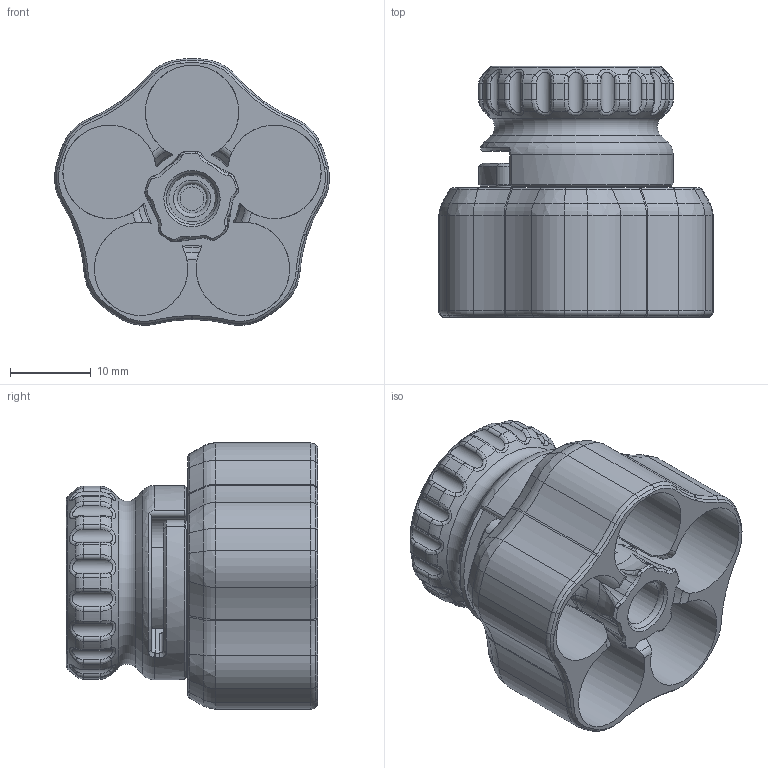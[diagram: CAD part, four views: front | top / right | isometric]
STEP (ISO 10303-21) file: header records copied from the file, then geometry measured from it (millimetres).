
FILE_DESCRIPTION(/* description */ (''),/* implementation_level */ '2;1');
FILE_NAME(/* name */ 'Speed Loader.step',/* time_stamp */ '2021-05-12T06:14:48-04:00',/* author */ (''),/* organization */ (''),/* preprocessor_version */ 'ST-DEVELOPER v18.1',/* originating_system */ 'Autodesk Translation Framework v10.6.0.1341',/* authorisation */ '');
FILE_SCHEMA (('AUTOMOTIVE_DESIGN { 1 0 10303 214 3 1 1 }'));
Length unit declared in the file: millimetre
Products named in the file (1): Speed Loader
Bounding box: 33.93 x 31 x 32.9 mm (x, y, z)
Volume: 11893.4 mm3; surface area: 8768.2 mm2
Topology: 3 solids, 3 shells, 729 faces, 1746 edges, 1012 vertices
Faces by surface type: bspline 219, cylinder 205, torus 143, cone 93, plane 64, sphere 5
Full cylindrical faces by diameter (mm): 2.9 x1, 3.6 x1, 3.7 x1, 5.75 x1, 8.75 x1, 9.1 x1, 9.3 x1, 10 x1, 16.6 x1, 18.6 x1
Entity records: 27437 total; most frequent: CARTESIAN_POINT 11790, ORIENTED_EDGE 3440, DIRECTION 3028, EDGE_CURVE 1720, AXIS2_PLACEMENT_3D 1302, VERTEX_POINT 1012, CIRCLE 791, EDGE_LOOP 748
